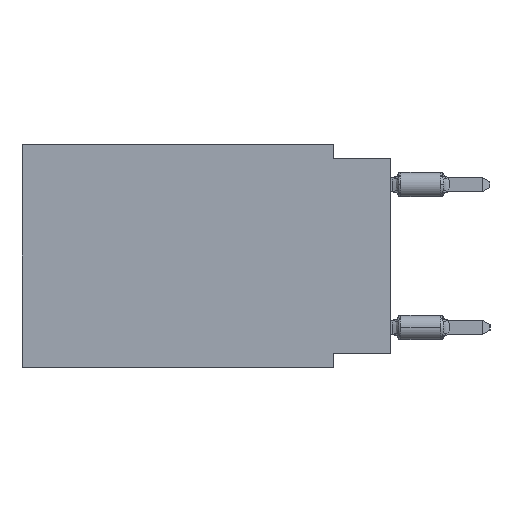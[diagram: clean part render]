
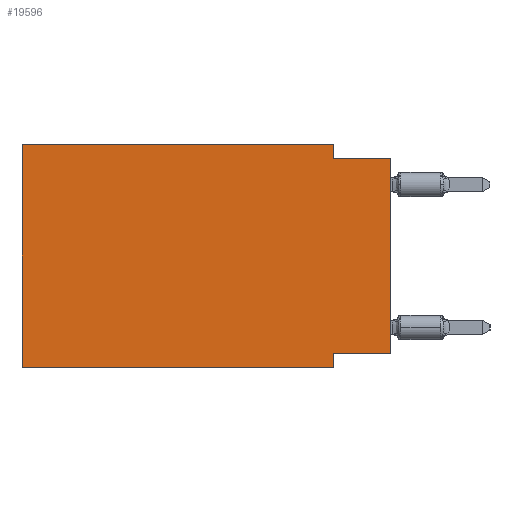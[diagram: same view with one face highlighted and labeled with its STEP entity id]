
A CAD part, left-side view. The second image highlights one B-rep face of the part: STEP entity #19596.
In plain terms, the highlighted planar face has unit normal (-1, 0, 0).
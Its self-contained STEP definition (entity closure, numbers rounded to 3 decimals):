
#13 = ORIENTED_EDGE ( 'NONE', *, *, #13459, .T. ) ;
#1419 = CARTESIAN_POINT ( 'NONE',  ( 0., 2.54, 0. ) ) ;
#2049 = ORIENTED_EDGE ( 'NONE', *, *, #2793, .T. ) ;
#2290 = VECTOR ( 'NONE', #9770, 1000. ) ;
#2520 = CARTESIAN_POINT ( 'NONE',  ( 0., 0., -9.271 ) ) ;
#2793 = EDGE_CURVE ( 'NONE', #5947, #2828, #14331, .T. ) ;
#2828 = VERTEX_POINT ( 'NONE', #7569 ) ;
#3064 = VERTEX_POINT ( 'NONE', #13596 ) ;
#3612 = EDGE_CURVE ( 'NONE', #3064, #19927, #14207, .T. ) ;
#3624 = CARTESIAN_POINT ( 'NONE',  ( 0., 16.383, 0. ) ) ;
#4664 = DIRECTION ( 'NONE',  ( 0., 0., 1. ) ) ;
#5170 = ORIENTED_EDGE ( 'NONE', *, *, #16020, .F. ) ;
#5792 = AXIS2_PLACEMENT_3D ( 'NONE', #23010, #25660, #8007 ) ;
#5887 = EDGE_CURVE ( 'NONE', #29654, #2828, #22956, .T. ) ;
#5947 = VERTEX_POINT ( 'NONE', #7939 ) ;
#6396 = DIRECTION ( 'NONE',  ( 0., -1., 0. ) ) ;
#6853 = ORIENTED_EDGE ( 'NONE', *, *, #24880, .F. ) ;
#6973 = CARTESIAN_POINT ( 'NONE',  ( 0., 16.383, 0. ) ) ;
#7569 = CARTESIAN_POINT ( 'NONE',  ( 0., 2.54, -9.906 ) ) ;
#7939 = CARTESIAN_POINT ( 'NONE',  ( 0., 16.383, -9.906 ) ) ;
#8003 = VECTOR ( 'NONE', #4664, 1000. ) ;
#8007 = DIRECTION ( 'NONE',  ( 0., 0., -1. ) ) ;
#8331 = PLANE ( 'NONE',  #5792 ) ;
#8568 = DIRECTION ( 'NONE',  ( 0., -1., 0. ) ) ;
#9162 = DIRECTION ( 'NONE',  ( 0., 0., -1. ) ) ;
#9770 = DIRECTION ( 'NONE',  ( 0., 0., 1. ) ) ;
#10476 = VECTOR ( 'NONE', #11577, 1000. ) ;
#10481 = FACE_OUTER_BOUND ( 'NONE', #19748, .T. ) ;
#10734 = LINE ( 'NONE', #18805, #15527 ) ;
#11577 = DIRECTION ( 'NONE',  ( 0., -1., 0. ) ) ;
#11750 = VERTEX_POINT ( 'NONE', #2520 ) ;
#11878 = CARTESIAN_POINT ( 'NONE',  ( 0., 16.383, -9.906 ) ) ;
#12403 = ORIENTED_EDGE ( 'NONE', *, *, #3612, .F. ) ;
#13206 = CARTESIAN_POINT ( 'NONE',  ( 0., 2.54, -9.906 ) ) ;
#13245 = VERTEX_POINT ( 'NONE', #24099 ) ;
#13459 = EDGE_CURVE ( 'NONE', #11750, #19927, #22599, .T. ) ;
#13514 = VERTEX_POINT ( 'NONE', #3624 ) ;
#13596 = CARTESIAN_POINT ( 'NONE',  ( 0., 2.54, -0.635 ) ) ;
#14131 = LINE ( 'NONE', #16955, #28510 ) ;
#14207 = LINE ( 'NONE', #26426, #10476 ) ;
#14331 = LINE ( 'NONE', #11878, #25773 ) ;
#14533 = VECTOR ( 'NONE', #9162, 1000. ) ;
#15527 = VECTOR ( 'NONE', #28854, 1000. ) ;
#15761 = ORIENTED_EDGE ( 'NONE', *, *, #23860, .F. ) ;
#16020 = EDGE_CURVE ( 'NONE', #11750, #29654, #10734, .T. ) ;
#16402 = ORIENTED_EDGE ( 'NONE', *, *, #5887, .F. ) ;
#16955 = CARTESIAN_POINT ( 'NONE',  ( 0., 16.383, 0. ) ) ;
#16968 = EDGE_CURVE ( 'NONE', #13245, #3064, #29590, .T. ) ;
#18805 = CARTESIAN_POINT ( 'NONE',  ( 0., 0., -9.271 ) ) ;
#19596 = ADVANCED_FACE ( 'NONE', ( #10481 ), #8331, .F. ) ;
#19748 = EDGE_LOOP ( 'NONE', ( #13, #12403, #23088, #15761, #6853, #2049, #16402, #5170 ) ) ;
#19927 = VERTEX_POINT ( 'NONE', #27700 ) ;
#19989 = VECTOR ( 'NONE', #20817, 1000. ) ;
#20817 = DIRECTION ( 'NONE',  ( 0., 0., -1. ) ) ;
#22471 = LINE ( 'NONE', #6973, #8003 ) ;
#22599 = LINE ( 'NONE', #30350, #2290 ) ;
#22956 = LINE ( 'NONE', #13206, #19989 ) ;
#23010 = CARTESIAN_POINT ( 'NONE',  ( 0., 16.383, 0. ) ) ;
#23088 = ORIENTED_EDGE ( 'NONE', *, *, #16968, .F. ) ;
#23860 = EDGE_CURVE ( 'NONE', #13514, #13245, #14131, .T. ) ;
#24099 = CARTESIAN_POINT ( 'NONE',  ( 0., 2.54, 0. ) ) ;
#24880 = EDGE_CURVE ( 'NONE', #5947, #13514, #22471, .T. ) ;
#24966 = CARTESIAN_POINT ( 'NONE',  ( 0., 2.54, -9.271 ) ) ;
#25660 = DIRECTION ( 'NONE',  ( 1., 0., 0. ) ) ;
#25773 = VECTOR ( 'NONE', #8568, 1000. ) ;
#26426 = CARTESIAN_POINT ( 'NONE',  ( 0., 0., -0.635 ) ) ;
#27700 = CARTESIAN_POINT ( 'NONE',  ( 0., 0., -0.635 ) ) ;
#28510 = VECTOR ( 'NONE', #6396, 1000. ) ;
#28854 = DIRECTION ( 'NONE',  ( 0., 1., 0. ) ) ;
#29590 = LINE ( 'NONE', #1419, #14533 ) ;
#29654 = VERTEX_POINT ( 'NONE', #24966 ) ;
#30350 = CARTESIAN_POINT ( 'NONE',  ( 0., 0., 0. ) ) ;
